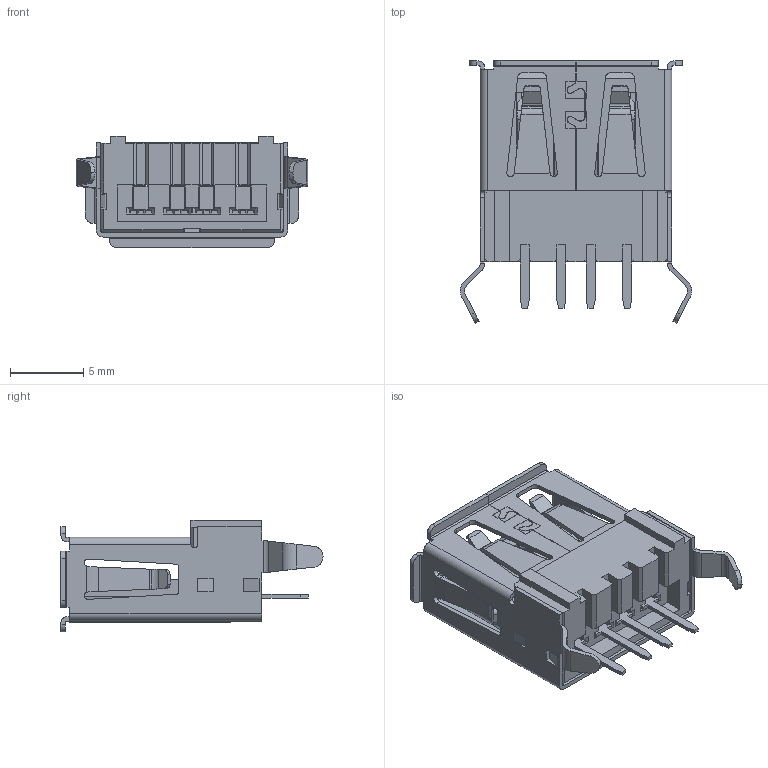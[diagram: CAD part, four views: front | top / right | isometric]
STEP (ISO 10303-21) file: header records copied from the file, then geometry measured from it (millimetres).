
FILE_DESCRIPTION (( 'STEP AP214' ), '1' );
FILE_NAME ('690E104-24C-421.STEP', '2021-01-14T12:40:00', ( '' ), ( '' ), 'SwSTEP 2.0', 'SolidWorks 2020', '' );
FILE_SCHEMA (( 'AUTOMOTIVE_DESIGN' ));
Length unit declared in the file: millimetre
Products named in the file (5): Contact 690E104-X4C-42X; Insulator 690E104-X4C-42X_Black; MYLAR 690E104-X4C-42X; Shell 690E104-X4C-42X; 690E104-24C-421
Assembly tree (7 placements, depth 2):
  690E104-24C-421
    Insulator 690E104-X4C-42X_Black
    Shell 690E104-X4C-42X
    Contact 690E104-X4C-42X  x4
    MYLAR 690E104-X4C-42X
Bounding box: 15.82 x 17.9 x 7.64 mm (x, y, z)
Volume: 571 mm3; surface area: 2136.9 mm2
Topology: 7 solids, 7 shells, 742 faces, 2124 edges, 1402 vertices
Faces by surface type: plane 558, cylinder 184
Entity records: 20292 total; most frequent: CARTESIAN_POINT 4968, ORIENTED_EDGE 3420, DIRECTION 2705, EDGE_CURVE 1710, VECTOR 1337, LINE 1337, VERTEX_POINT 1126, AXIS2_PLACEMENT_3D 684
